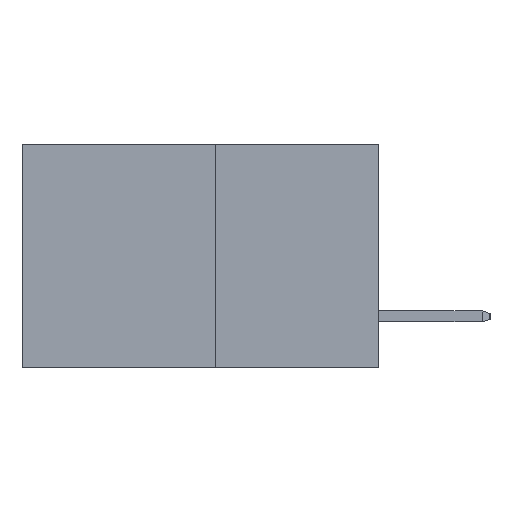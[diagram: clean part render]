
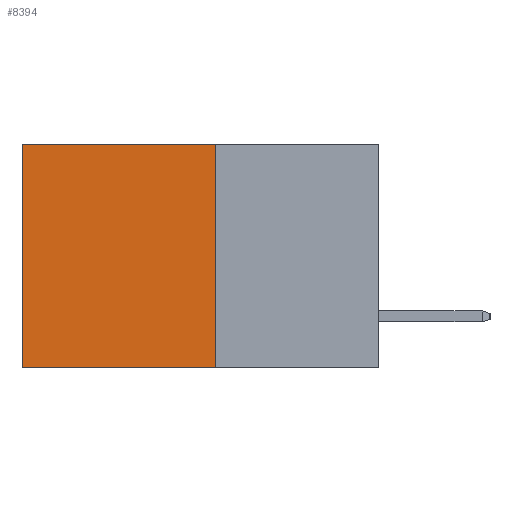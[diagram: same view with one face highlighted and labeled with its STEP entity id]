
A CAD part, left-side view. The second image highlights one B-rep face of the part: STEP entity #8394.
In plain terms, the highlighted planar face has unit normal (-1, 0, 0).
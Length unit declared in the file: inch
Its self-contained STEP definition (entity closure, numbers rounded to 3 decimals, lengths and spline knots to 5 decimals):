
#5 = DIRECTION ( 'NONE',  ( 0., 1., 0. ) ) ;
#172 = DIRECTION ( 'NONE',  ( 0., 0., -1. ) ) ;
#338 = VECTOR ( 'NONE', #5, 39.37008 ) ;
#508 = CARTESIAN_POINT ( 'NONE',  ( 0.277, 0.27, 0. ) ) ;
#900 = LINE ( 'NONE', #9443, #9958 ) ;
#1138 = VERTEX_POINT ( 'NONE', #7510 ) ;
#1375 = ORIENTED_EDGE ( 'NONE', *, *, #2614, .F. ) ;
#2086 = FACE_OUTER_BOUND ( 'NONE', #3907, .T. ) ;
#2118 = CARTESIAN_POINT ( 'NONE',  ( 0.277, 0.27, -0.37 ) ) ;
#2614 = EDGE_CURVE ( 'NONE', #1138, #10887, #900, .T. ) ;
#3009 = VECTOR ( 'NONE', #4768, 39.37008 ) ;
#3186 = DIRECTION ( 'NONE',  ( 0., 0., -1. ) ) ;
#3631 = EDGE_CURVE ( 'NONE', #9285, #1138, #4582, .T. ) ;
#3748 = ORIENTED_EDGE ( 'NONE', *, *, #3631, .F. ) ;
#3907 = EDGE_LOOP ( 'NONE', ( #5882, #1375, #3748, #6146 ) ) ;
#4582 = LINE ( 'NONE', #5607, #9189 ) ;
#4768 = DIRECTION ( 'NONE',  ( 0., 0., -1. ) ) ;
#5233 = DIRECTION ( 'NONE',  ( 0., 1., 0. ) ) ;
#5442 = LINE ( 'NONE', #6503, #3009 ) ;
#5541 = CARTESIAN_POINT ( 'NONE',  ( 0.277, 0.59, -0.37 ) ) ;
#5607 = CARTESIAN_POINT ( 'NONE',  ( 0.277, 0.27, -0.37 ) ) ;
#5659 = CARTESIAN_POINT ( 'NONE',  ( 0.277, 0.59, 0. ) ) ;
#5882 = ORIENTED_EDGE ( 'NONE', *, *, #11023, .T. ) ;
#6146 = ORIENTED_EDGE ( 'NONE', *, *, #6330, .T. ) ;
#6241 = DIRECTION ( 'NONE',  ( 1., 0., 0. ) ) ;
#6330 = EDGE_CURVE ( 'NONE', #9285, #7568, #10259, .T. ) ;
#6503 = CARTESIAN_POINT ( 'NONE',  ( 0.277, 0.59, -0.37 ) ) ;
#7087 = AXIS2_PLACEMENT_3D ( 'NONE', #2118, #6241, #172 ) ;
#7510 = CARTESIAN_POINT ( 'NONE',  ( 0.277, 0.27, -0.37 ) ) ;
#7568 = VERTEX_POINT ( 'NONE', #5659 ) ;
#8394 = ADVANCED_FACE ( 'NONE', ( #2086 ), #10810, .F. ) ;
#9052 = CARTESIAN_POINT ( 'NONE',  ( 0.277, 0.27, 0. ) ) ;
#9189 = VECTOR ( 'NONE', #3186, 39.37008 ) ;
#9285 = VERTEX_POINT ( 'NONE', #9052 ) ;
#9443 = CARTESIAN_POINT ( 'NONE',  ( 0.277, 0.27, -0.37 ) ) ;
#9958 = VECTOR ( 'NONE', #5233, 39.37008 ) ;
#10259 = LINE ( 'NONE', #508, #338 ) ;
#10810 = PLANE ( 'NONE',  #7087 ) ;
#10887 = VERTEX_POINT ( 'NONE', #5541 ) ;
#11023 = EDGE_CURVE ( 'NONE', #7568, #10887, #5442, .T. ) ;
